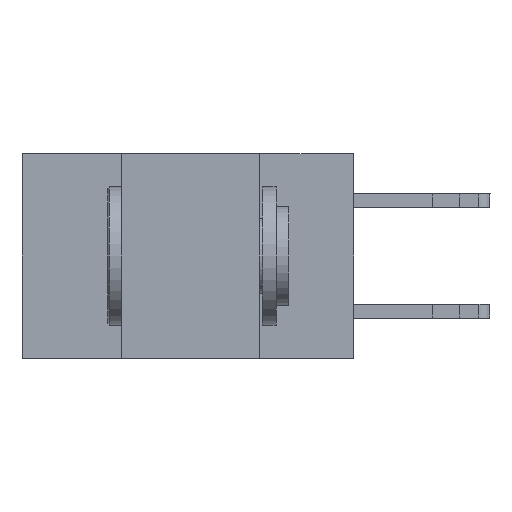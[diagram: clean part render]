
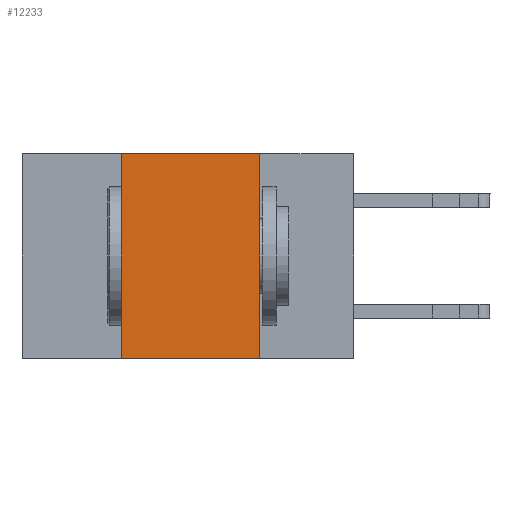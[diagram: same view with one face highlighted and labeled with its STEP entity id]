
A CAD part, left-side view. The second image highlights one B-rep face of the part: STEP entity #12233.
In plain terms, the highlighted planar face has unit normal (-1, 0, 0).
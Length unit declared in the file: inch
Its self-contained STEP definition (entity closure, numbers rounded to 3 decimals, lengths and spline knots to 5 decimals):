
#204 = LINE ( 'NONE', #8385, #13835 ) ;
#1666 = DIRECTION ( 'NONE',  ( 0., -1., 0. ) ) ;
#2058 = LINE ( 'NONE', #23792, #2318 ) ;
#2318 = VECTOR ( 'NONE', #1666, 39.37008 ) ;
#2708 = DIRECTION ( 'NONE',  ( 0., -1., 0. ) ) ;
#2939 = CARTESIAN_POINT ( 'NONE',  ( 0., 0.17, -0.37 ) ) ;
#3282 = VERTEX_POINT ( 'NONE', #21811 ) ;
#3766 = EDGE_CURVE ( 'NONE', #3282, #4330, #2058, .T. ) ;
#4330 = VERTEX_POINT ( 'NONE', #10934 ) ;
#4469 = ORIENTED_EDGE ( 'NONE', *, *, #11828, .F. ) ;
#4760 = VERTEX_POINT ( 'NONE', #2939 ) ;
#5700 = AXIS2_PLACEMENT_3D ( 'NONE', #16210, #10737, #23651 ) ;
#7860 = VECTOR ( 'NONE', #10655, 39.37008 ) ;
#7907 = VECTOR ( 'NONE', #21751, 39.37008 ) ;
#8279 = EDGE_CURVE ( 'NONE', #16074, #4760, #204, .T. ) ;
#8385 = CARTESIAN_POINT ( 'NONE',  ( 0., 0.6, -0.37 ) ) ;
#8507 = CARTESIAN_POINT ( 'NONE',  ( 0., 0.42, -0.37 ) ) ;
#10655 = DIRECTION ( 'NONE',  ( 0., 0., -1. ) ) ;
#10737 = DIRECTION ( 'NONE',  ( 1., 0., 0. ) ) ;
#10934 = CARTESIAN_POINT ( 'NONE',  ( 0., 0.17, 0. ) ) ;
#11828 = EDGE_CURVE ( 'NONE', #4330, #4760, #22620, .T. ) ;
#11995 = EDGE_LOOP ( 'NONE', ( #4469, #14097, #19820, #21368 ) ) ;
#12233 = ADVANCED_FACE ( 'NONE', ( #16236 ), #18026, .F. ) ;
#13835 = VECTOR ( 'NONE', #2708, 39.37008 ) ;
#14097 = ORIENTED_EDGE ( 'NONE', *, *, #3766, .F. ) ;
#16074 = VERTEX_POINT ( 'NONE', #8507 ) ;
#16171 = CARTESIAN_POINT ( 'NONE',  ( 0., 0.42, 0. ) ) ;
#16210 = CARTESIAN_POINT ( 'NONE',  ( 0., 0.6, 0. ) ) ;
#16236 = FACE_OUTER_BOUND ( 'NONE', #11995, .T. ) ;
#18026 = PLANE ( 'NONE',  #5700 ) ;
#18356 = LINE ( 'NONE', #16171, #7907 ) ;
#19111 = EDGE_CURVE ( 'NONE', #16074, #3282, #18356, .T. ) ;
#19820 = ORIENTED_EDGE ( 'NONE', *, *, #19111, .F. ) ;
#21368 = ORIENTED_EDGE ( 'NONE', *, *, #8279, .T. ) ;
#21751 = DIRECTION ( 'NONE',  ( 0., 0., 1. ) ) ;
#21811 = CARTESIAN_POINT ( 'NONE',  ( 0., 0.42, 0. ) ) ;
#22620 = LINE ( 'NONE', #23647, #7860 ) ;
#23647 = CARTESIAN_POINT ( 'NONE',  ( 0., 0.17, 0. ) ) ;
#23651 = DIRECTION ( 'NONE',  ( 0., 0., -1. ) ) ;
#23792 = CARTESIAN_POINT ( 'NONE',  ( 0., 0.6, 0. ) ) ;
